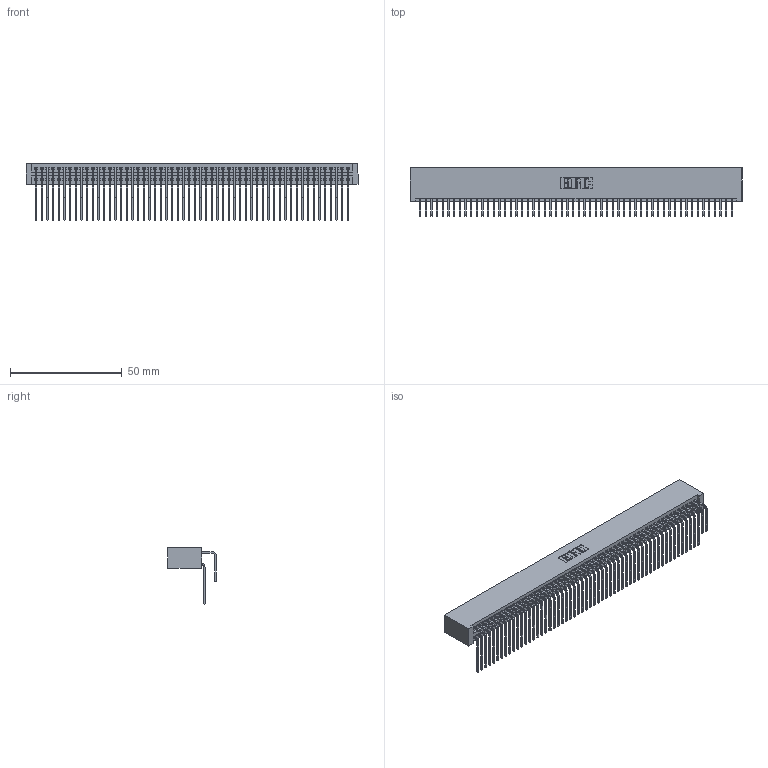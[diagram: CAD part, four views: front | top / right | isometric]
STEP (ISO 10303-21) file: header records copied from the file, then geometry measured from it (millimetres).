
FILE_DESCRIPTION (( 'STEP AP203' ), '1' );
FILE_NAME ('345-112-558-201.STEP', '2019-11-04T23:19:51', ( '' ), ( '' ), 'SwSTEP 2.0', 'SolidWorks 2016', '' );
FILE_SCHEMA (( 'CONFIG_CONTROL_DESIGN' ));
Length unit declared in the file: inch
Products named in the file (4): 345 Part_No Mounting Lugs; 345-112-558-201; 345-292-001_558 559 Tail - 1; 345-292-001_558 Tail - 2
Assembly tree (113 placements, depth 2):
  345-112-558-201
    345 Part_No Mounting Lugs
    345-292-001_558 559 Tail - 1  x56
    345-292-001_558 Tail - 2  x56
Bounding box: 148.84 x 21.83 x 25.53 mm (x, y, z)
Volume: 15850.8 mm3; surface area: 27042.8 mm2
Topology: 113 solids, 113 shells, 5942 faces, 17677 edges, 11634 vertices
Faces by surface type: plane 3996, cylinder 1946
Entity records: 43429 total; most frequent: CARTESIAN_POINT 7311, ORIENTED_EDGE 7194, DIRECTION 6397, EDGE_CURVE 3597, VECTOR 3209, LINE 3209, VERTEX_POINT 2394, AXIS2_PLACEMENT_3D 1594
